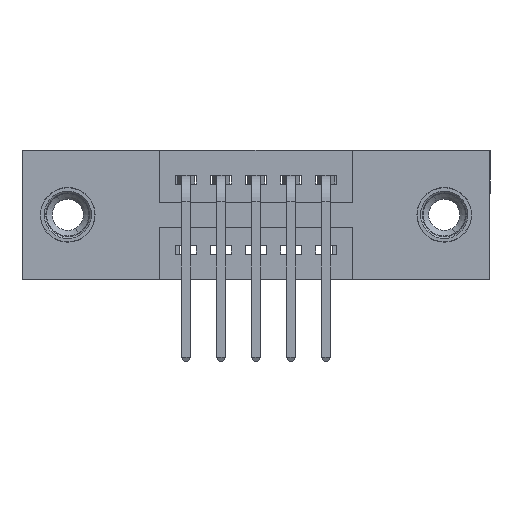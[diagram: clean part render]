
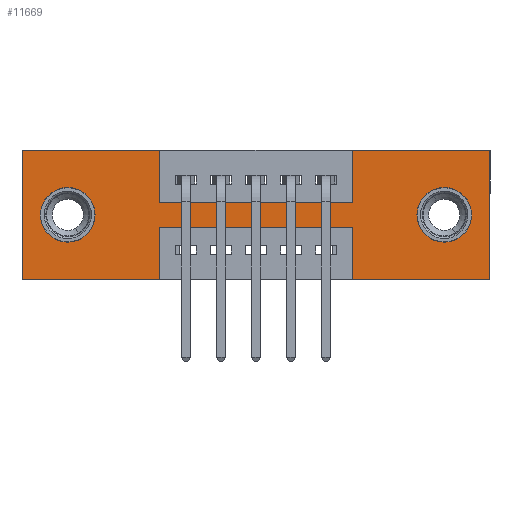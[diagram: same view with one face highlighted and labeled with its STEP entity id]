
A CAD part, front view. The second image highlights one B-rep face of the part: STEP entity #11669.
In plain terms, the highlighted planar face has unit normal (0, -1, 0).
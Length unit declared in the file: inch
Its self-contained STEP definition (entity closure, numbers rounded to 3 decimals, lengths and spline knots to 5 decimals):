
#108 = CARTESIAN_POINT ( 'NONE',  ( 1.335, 0., 0. ) ) ;
#134 = DIRECTION ( 'NONE',  ( 1., 0., 0. ) ) ;
#284 = DIRECTION ( 'NONE',  ( 0., 0., -1. ) ) ;
#789 = VECTOR ( 'NONE', #3667, 39.37008 ) ;
#954 = VECTOR ( 'NONE', #284, 39.37008 ) ;
#987 = DIRECTION ( 'NONE',  ( 0., -1., 0. ) ) ;
#1069 = LINE ( 'NONE', #1931, #5986 ) ;
#1078 = VECTOR ( 'NONE', #4020, 39.37008 ) ;
#1084 = CARTESIAN_POINT ( 'NONE',  ( 0., 0., 0. ) ) ;
#1143 = EDGE_CURVE ( 'NONE', #3493, #7531, #12961, .T. ) ;
#1381 = CIRCLE ( 'NONE', #8469, 0.078 ) ;
#1429 = LINE ( 'NONE', #7269, #9722 ) ;
#1532 = VERTEX_POINT ( 'NONE', #7872 ) ;
#1587 = LINE ( 'NONE', #6936, #13032 ) ;
#1628 = LINE ( 'NONE', #6237, #9923 ) ;
#1905 = VERTEX_POINT ( 'NONE', #11495 ) ;
#1931 = CARTESIAN_POINT ( 'NONE',  ( 0.9425, 0., -0.37 ) ) ;
#1951 = VERTEX_POINT ( 'NONE', #108 ) ;
#2047 = CARTESIAN_POINT ( 'NONE',  ( 1.205, 0., -0.185 ) ) ;
#2084 = LINE ( 'NONE', #10248, #1078 ) ;
#2137 = DIRECTION ( 'NONE',  ( 1., 0., 0. ) ) ;
#2237 = ORIENTED_EDGE ( 'NONE', *, *, #7620, .F. ) ;
#2371 = DIRECTION ( 'NONE',  ( 0., 0., -1. ) ) ;
#2453 = CARTESIAN_POINT ( 'NONE',  ( 0.3925, 0., 0. ) ) ;
#2477 = FACE_BOUND ( 'NONE', #5376, .T. ) ;
#2483 = ORIENTED_EDGE ( 'NONE', *, *, #1143, .T. ) ;
#2641 = DIRECTION ( 'NONE',  ( 0., 1., 0. ) ) ;
#2644 = DIRECTION ( 'NONE',  ( -1., 0., 0. ) ) ;
#2726 = EDGE_CURVE ( 'NONE', #1951, #13336, #9121, .T. ) ;
#3025 = CARTESIAN_POINT ( 'NONE',  ( 0., 0., 0. ) ) ;
#3033 = ORIENTED_EDGE ( 'NONE', *, *, #5980, .T. ) ;
#3175 = VECTOR ( 'NONE', #2644, 39.37008 ) ;
#3256 = DIRECTION ( 'NONE',  ( 0., 1., 0. ) ) ;
#3466 = EDGE_CURVE ( 'NONE', #11132, #4399, #1628, .T. ) ;
#3493 = VERTEX_POINT ( 'NONE', #8403 ) ;
#3495 = CARTESIAN_POINT ( 'NONE',  ( 0.9425, 0., 0. ) ) ;
#3667 = DIRECTION ( 'NONE',  ( 0., 0., -1. ) ) ;
#3745 = CARTESIAN_POINT ( 'NONE',  ( 0.3925, 0., -0.15 ) ) ;
#3759 = LINE ( 'NONE', #6584, #954 ) ;
#3842 = DIRECTION ( 'NONE',  ( 0., 1., 0. ) ) ;
#4020 = DIRECTION ( 'NONE',  ( -1., 0., 0. ) ) ;
#4131 = DIRECTION ( 'NONE',  ( 1., 0., 0. ) ) ;
#4180 = DIRECTION ( 'NONE',  ( 0., 0., 1. ) ) ;
#4354 = CARTESIAN_POINT ( 'NONE',  ( 0., 0., 0. ) ) ;
#4399 = VERTEX_POINT ( 'NONE', #2453 ) ;
#4612 = CARTESIAN_POINT ( 'NONE',  ( 0.3925, 0., -0.37 ) ) ;
#4726 = EDGE_CURVE ( 'NONE', #10475, #11529, #1429, .T. ) ;
#4883 = VERTEX_POINT ( 'NONE', #4612 ) ;
#5024 = EDGE_LOOP ( 'NONE', ( #10161, #12556, #12971, #2237, #5735, #5534, #5718, #8345, #10811, #8012, #6880, #12675 ) ) ;
#5099 = EDGE_CURVE ( 'NONE', #1905, #7440, #8253, .T. ) ;
#5263 = EDGE_CURVE ( 'NONE', #1532, #6128, #1069, .T. ) ;
#5266 = FACE_BOUND ( 'NONE', #10201, .T. ) ;
#5376 = EDGE_LOOP ( 'NONE', ( #3033, #6021 ) ) ;
#5482 = DIRECTION ( 'NONE',  ( 0., 1., 0. ) ) ;
#5534 = ORIENTED_EDGE ( 'NONE', *, *, #11779, .F. ) ;
#5624 = LINE ( 'NONE', #1084, #10820 ) ;
#5659 = CARTESIAN_POINT ( 'NONE',  ( 0.9425, 0., -0.22 ) ) ;
#5718 = ORIENTED_EDGE ( 'NONE', *, *, #6874, .F. ) ;
#5735 = ORIENTED_EDGE ( 'NONE', *, *, #2726, .F. ) ;
#5752 = ORIENTED_EDGE ( 'NONE', *, *, #9525, .T. ) ;
#5768 = AXIS2_PLACEMENT_3D ( 'NONE', #11692, #5482, #12776 ) ;
#5856 = CARTESIAN_POINT ( 'NONE',  ( 0.3925, 0., -0.22 ) ) ;
#5869 = CARTESIAN_POINT ( 'NONE',  ( 0.9425, 0., -0.15 ) ) ;
#5980 = EDGE_CURVE ( 'NONE', #7440, #1905, #11322, .T. ) ;
#5986 = VECTOR ( 'NONE', #8202, 39.37008 ) ;
#6021 = ORIENTED_EDGE ( 'NONE', *, *, #5099, .T. ) ;
#6128 = VERTEX_POINT ( 'NONE', #5659 ) ;
#6205 = EDGE_CURVE ( 'NONE', #4883, #11846, #8708, .T. ) ;
#6216 = PLANE ( 'NONE',  #9976 ) ;
#6237 = CARTESIAN_POINT ( 'NONE',  ( 0., 0., 0. ) ) ;
#6584 = CARTESIAN_POINT ( 'NONE',  ( 0.3925, 0., 0. ) ) ;
#6719 = LINE ( 'NONE', #4354, #11921 ) ;
#6763 = LINE ( 'NONE', #9399, #13213 ) ;
#6874 = EDGE_CURVE ( 'NONE', #11529, #8049, #6763, .T. ) ;
#6880 = ORIENTED_EDGE ( 'NONE', *, *, #10136, .F. ) ;
#6936 = CARTESIAN_POINT ( 'NONE',  ( 0., 0., -0.37 ) ) ;
#7269 = CARTESIAN_POINT ( 'NONE',  ( 0.3925, 0., -0.15 ) ) ;
#7419 = EDGE_CURVE ( 'NONE', #6128, #9486, #2084, .T. ) ;
#7440 = VERTEX_POINT ( 'NONE', #8245 ) ;
#7531 = VERTEX_POINT ( 'NONE', #10615 ) ;
#7560 = CARTESIAN_POINT ( 'NONE',  ( 0., 0., -0.37 ) ) ;
#7620 = EDGE_CURVE ( 'NONE', #13336, #1532, #1587, .T. ) ;
#7800 = CARTESIAN_POINT ( 'NONE',  ( 1.335, 0., 0. ) ) ;
#7872 = CARTESIAN_POINT ( 'NONE',  ( 0.9425, 0., -0.37 ) ) ;
#8012 = ORIENTED_EDGE ( 'NONE', *, *, #3466, .F. ) ;
#8049 = VERTEX_POINT ( 'NONE', #3495 ) ;
#8179 = CARTESIAN_POINT ( 'NONE',  ( 1.335, 0., -0.37 ) ) ;
#8202 = DIRECTION ( 'NONE',  ( 0., 0., 1. ) ) ;
#8245 = CARTESIAN_POINT ( 'NONE',  ( 0.13, 0., -0.107 ) ) ;
#8253 = CIRCLE ( 'NONE', #10008, 0.078 ) ;
#8293 = DIRECTION ( 'NONE',  ( 0., 0., -1. ) ) ;
#8345 = ORIENTED_EDGE ( 'NONE', *, *, #4726, .F. ) ;
#8403 = CARTESIAN_POINT ( 'NONE',  ( 1.205, 0., -0.263 ) ) ;
#8469 = AXIS2_PLACEMENT_3D ( 'NONE', #9485, #3256, #10536 ) ;
#8708 = LINE ( 'NONE', #9909, #3175 ) ;
#8850 = AXIS2_PLACEMENT_3D ( 'NONE', #2047, #2641, #2371 ) ;
#9121 = LINE ( 'NONE', #7800, #789 ) ;
#9286 = CARTESIAN_POINT ( 'NONE',  ( 0., 0., -0.37 ) ) ;
#9399 = CARTESIAN_POINT ( 'NONE',  ( 0.9425, 0., 0. ) ) ;
#9485 = CARTESIAN_POINT ( 'NONE',  ( 1.205, 0., -0.185 ) ) ;
#9486 = VERTEX_POINT ( 'NONE', #5856 ) ;
#9525 = EDGE_CURVE ( 'NONE', #7531, #3493, #1381, .T. ) ;
#9722 = VECTOR ( 'NONE', #4131, 39.37008 ) ;
#9909 = CARTESIAN_POINT ( 'NONE',  ( 0., 0., -0.37 ) ) ;
#9923 = VECTOR ( 'NONE', #2137, 39.37008 ) ;
#9976 = AXIS2_PLACEMENT_3D ( 'NONE', #9286, #987, #8293 ) ;
#10008 = AXIS2_PLACEMENT_3D ( 'NONE', #10072, #3842, #11125 ) ;
#10072 = CARTESIAN_POINT ( 'NONE',  ( 0.13, 0., -0.185 ) ) ;
#10136 = EDGE_CURVE ( 'NONE', #11846, #11132, #5624, .T. ) ;
#10161 = ORIENTED_EDGE ( 'NONE', *, *, #10983, .F. ) ;
#10201 = EDGE_LOOP ( 'NONE', ( #5752, #2483 ) ) ;
#10248 = CARTESIAN_POINT ( 'NONE',  ( 0.3925, 0., -0.22 ) ) ;
#10475 = VERTEX_POINT ( 'NONE', #3745 ) ;
#10536 = DIRECTION ( 'NONE',  ( 0., 0., -1. ) ) ;
#10615 = CARTESIAN_POINT ( 'NONE',  ( 1.205, 0., -0.107 ) ) ;
#10811 = ORIENTED_EDGE ( 'NONE', *, *, #12585, .F. ) ;
#10820 = VECTOR ( 'NONE', #11520, 39.37008 ) ;
#10983 = EDGE_CURVE ( 'NONE', #9486, #4883, #13451, .T. ) ;
#11003 = DIRECTION ( 'NONE',  ( 0., 0., -1. ) ) ;
#11109 = DIRECTION ( 'NONE',  ( -1., 0., 0. ) ) ;
#11125 = DIRECTION ( 'NONE',  ( 0., 0., 1. ) ) ;
#11132 = VERTEX_POINT ( 'NONE', #3025 ) ;
#11322 = CIRCLE ( 'NONE', #5768, 0.078 ) ;
#11495 = CARTESIAN_POINT ( 'NONE',  ( 0.13, 0., -0.263 ) ) ;
#11520 = DIRECTION ( 'NONE',  ( 0., 0., 1. ) ) ;
#11529 = VERTEX_POINT ( 'NONE', #5869 ) ;
#11669 = ADVANCED_FACE ( 'NONE', ( #5266, #2477, #13266 ), #6216, .T. ) ;
#11692 = CARTESIAN_POINT ( 'NONE',  ( 0.13, 0., -0.185 ) ) ;
#11779 = EDGE_CURVE ( 'NONE', #8049, #1951, #6719, .T. ) ;
#11846 = VERTEX_POINT ( 'NONE', #7560 ) ;
#11921 = VECTOR ( 'NONE', #134, 39.37008 ) ;
#12556 = ORIENTED_EDGE ( 'NONE', *, *, #7419, .F. ) ;
#12585 = EDGE_CURVE ( 'NONE', #4399, #10475, #3759, .T. ) ;
#12675 = ORIENTED_EDGE ( 'NONE', *, *, #6205, .F. ) ;
#12776 = DIRECTION ( 'NONE',  ( 0., 0., 1. ) ) ;
#12792 = VECTOR ( 'NONE', #11003, 39.37008 ) ;
#12961 = CIRCLE ( 'NONE', #8850, 0.078 ) ;
#12971 = ORIENTED_EDGE ( 'NONE', *, *, #5263, .F. ) ;
#13032 = VECTOR ( 'NONE', #11109, 39.37008 ) ;
#13148 = CARTESIAN_POINT ( 'NONE',  ( 0.3925, 0., -0.37 ) ) ;
#13213 = VECTOR ( 'NONE', #4180, 39.37008 ) ;
#13266 = FACE_OUTER_BOUND ( 'NONE', #5024, .T. ) ;
#13336 = VERTEX_POINT ( 'NONE', #8179 ) ;
#13451 = LINE ( 'NONE', #13148, #12792 ) ;
